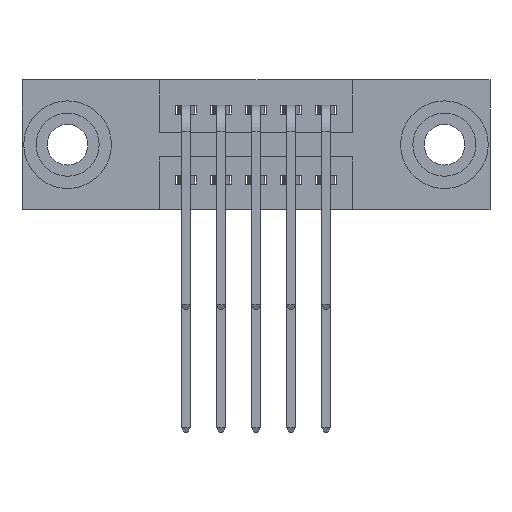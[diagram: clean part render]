
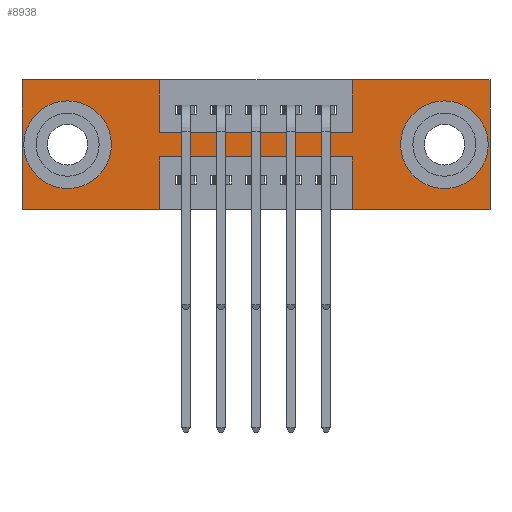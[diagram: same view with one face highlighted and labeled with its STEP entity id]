
A CAD part, front view. The second image highlights one B-rep face of the part: STEP entity #8938.
In plain terms, the highlighted planar face has unit normal (0, -1, 0).
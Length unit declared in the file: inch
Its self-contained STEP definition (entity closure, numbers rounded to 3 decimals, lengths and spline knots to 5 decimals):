
#132 = VECTOR ( 'NONE', #8937, 39.37008 ) ;
#180 = CARTESIAN_POINT ( 'NONE',  ( 0.13, 0., -0.107 ) ) ;
#190 = VERTEX_POINT ( 'NONE', #2204 ) ;
#202 = ORIENTED_EDGE ( 'NONE', *, *, #2390, .F. ) ;
#289 = LINE ( 'NONE', #6771, #3451 ) ;
#338 = CARTESIAN_POINT ( 'NONE',  ( 1.205, 0., -0.263 ) ) ;
#362 = VECTOR ( 'NONE', #2451, 39.37008 ) ;
#378 = EDGE_LOOP ( 'NONE', ( #10536, #8988 ) ) ;
#454 = CARTESIAN_POINT ( 'NONE',  ( 0.3925, 0., 0. ) ) ;
#638 = EDGE_CURVE ( 'NONE', #7686, #3815, #10066, .T. ) ;
#700 = LINE ( 'NONE', #9389, #9630 ) ;
#830 = CARTESIAN_POINT ( 'NONE',  ( 1.205, 0., -0.185 ) ) ;
#831 = LINE ( 'NONE', #9449, #10295 ) ;
#842 = EDGE_CURVE ( 'NONE', #7530, #3438, #9108, .T. ) ;
#853 = DIRECTION ( 'NONE',  ( -1., 0., 0. ) ) ;
#1065 = LINE ( 'NONE', #1571, #362 ) ;
#1109 = VERTEX_POINT ( 'NONE', #6565 ) ;
#1244 = VECTOR ( 'NONE', #3058, 39.37008 ) ;
#1246 = ORIENTED_EDGE ( 'NONE', *, *, #2250, .T. ) ;
#1366 = DIRECTION ( 'NONE',  ( 0., 1., 0. ) ) ;
#1538 = EDGE_CURVE ( 'NONE', #1109, #5867, #289, .T. ) ;
#1571 = CARTESIAN_POINT ( 'NONE',  ( 0., 0., 0. ) ) ;
#1738 = CARTESIAN_POINT ( 'NONE',  ( 0., 0., 0. ) ) ;
#1901 = EDGE_CURVE ( 'NONE', #7118, #190, #700, .T. ) ;
#1912 = CARTESIAN_POINT ( 'NONE',  ( 0.3925, 0., 0. ) ) ;
#2017 = AXIS2_PLACEMENT_3D ( 'NONE', #9764, #1366, #9196 ) ;
#2029 = CIRCLE ( 'NONE', #9321, 0.078 ) ;
#2113 = CARTESIAN_POINT ( 'NONE',  ( 0.3925, 0., -0.15 ) ) ;
#2202 = EDGE_CURVE ( 'NONE', #190, #5864, #2765, .T. ) ;
#2204 = CARTESIAN_POINT ( 'NONE',  ( 0.9425, 0., -0.37 ) ) ;
#2250 = EDGE_CURVE ( 'NONE', #8171, #9735, #3014, .T. ) ;
#2390 = EDGE_CURVE ( 'NONE', #4055, #7118, #831, .T. ) ;
#2399 = CARTESIAN_POINT ( 'NONE',  ( 0., 0., 0. ) ) ;
#2451 = DIRECTION ( 'NONE',  ( 1., 0., 0. ) ) ;
#2468 = DIRECTION ( 'NONE',  ( 0., 1., 0. ) ) ;
#2560 = FACE_OUTER_BOUND ( 'NONE', #3267, .T. ) ;
#2689 = VECTOR ( 'NONE', #5883, 39.37008 ) ;
#2765 = LINE ( 'NONE', #6328, #132 ) ;
#2874 = CARTESIAN_POINT ( 'NONE',  ( 0.3925, 0., -0.22 ) ) ;
#2914 = CARTESIAN_POINT ( 'NONE',  ( 0.3925, 0., -0.15 ) ) ;
#3014 = CIRCLE ( 'NONE', #3895, 0.078 ) ;
#3042 = CARTESIAN_POINT ( 'NONE',  ( 0., 0., -0.37 ) ) ;
#3047 = ORIENTED_EDGE ( 'NONE', *, *, #638, .F. ) ;
#3054 = CARTESIAN_POINT ( 'NONE',  ( 0.3925, 0., -0.22 ) ) ;
#3058 = DIRECTION ( 'NONE',  ( 1., 0., 0. ) ) ;
#3183 = VERTEX_POINT ( 'NONE', #2914 ) ;
#3197 = DIRECTION ( 'NONE',  ( -1., 0., 0. ) ) ;
#3214 = EDGE_CURVE ( 'NONE', #5265, #10917, #5685, .T. ) ;
#3267 = EDGE_LOOP ( 'NONE', ( #3047, #7719, #7498, #3424, #202, #5634, #7673, #6464, #8298, #10031, #10644, #8394 ) ) ;
#3424 = ORIENTED_EDGE ( 'NONE', *, *, #1901, .F. ) ;
#3438 = VERTEX_POINT ( 'NONE', #338 ) ;
#3451 = VECTOR ( 'NONE', #5842, 39.37008 ) ;
#3535 = EDGE_CURVE ( 'NONE', #3807, #3183, #10944, .T. ) ;
#3540 = VECTOR ( 'NONE', #8342, 39.37008 ) ;
#3636 = CARTESIAN_POINT ( 'NONE',  ( 0.13, 0., -0.185 ) ) ;
#3680 = ORIENTED_EDGE ( 'NONE', *, *, #3994, .T. ) ;
#3701 = EDGE_CURVE ( 'NONE', #5867, #4055, #1065, .T. ) ;
#3708 = DIRECTION ( 'NONE',  ( 0., 1., 0. ) ) ;
#3807 = VERTEX_POINT ( 'NONE', #1912 ) ;
#3815 = VERTEX_POINT ( 'NONE', #5576 ) ;
#3895 = AXIS2_PLACEMENT_3D ( 'NONE', #7612, #2468, #5875 ) ;
#3994 = EDGE_CURVE ( 'NONE', #9735, #8171, #2029, .T. ) ;
#4020 = CARTESIAN_POINT ( 'NONE',  ( 0.3925, 0., -0.37 ) ) ;
#4055 = VERTEX_POINT ( 'NONE', #9660 ) ;
#4200 = DIRECTION ( 'NONE',  ( 0., 1., 0. ) ) ;
#4464 = LINE ( 'NONE', #6498, #10279 ) ;
#4509 = AXIS2_PLACEMENT_3D ( 'NONE', #3042, #4632, #10741 ) ;
#4632 = DIRECTION ( 'NONE',  ( 0., -1., 0. ) ) ;
#5265 = VERTEX_POINT ( 'NONE', #6863 ) ;
#5469 = VECTOR ( 'NONE', #5832, 39.37008 ) ;
#5576 = CARTESIAN_POINT ( 'NONE',  ( 0.3925, 0., -0.37 ) ) ;
#5630 = EDGE_CURVE ( 'NONE', #3183, #1109, #10305, .T. ) ;
#5634 = ORIENTED_EDGE ( 'NONE', *, *, #3701, .F. ) ;
#5685 = LINE ( 'NONE', #10138, #10539 ) ;
#5832 = DIRECTION ( 'NONE',  ( 0., 0., -1. ) ) ;
#5842 = DIRECTION ( 'NONE',  ( 0., 0., 1. ) ) ;
#5864 = VERTEX_POINT ( 'NONE', #7512 ) ;
#5867 = VERTEX_POINT ( 'NONE', #6929 ) ;
#5875 = DIRECTION ( 'NONE',  ( 0., 0., 1. ) ) ;
#5876 = DIRECTION ( 'NONE',  ( 0., 0., -1. ) ) ;
#5883 = DIRECTION ( 'NONE',  ( 1., 0., 0. ) ) ;
#6102 = EDGE_CURVE ( 'NONE', #3438, #7530, #10172, .T. ) ;
#6198 = DIRECTION ( 'NONE',  ( 0., 0., 1. ) ) ;
#6328 = CARTESIAN_POINT ( 'NONE',  ( 0.9425, 0., -0.37 ) ) ;
#6416 = AXIS2_PLACEMENT_3D ( 'NONE', #830, #4200, #5876 ) ;
#6464 = ORIENTED_EDGE ( 'NONE', *, *, #5630, .F. ) ;
#6498 = CARTESIAN_POINT ( 'NONE',  ( 0., 0., -0.37 ) ) ;
#6565 = CARTESIAN_POINT ( 'NONE',  ( 0.9425, 0., -0.15 ) ) ;
#6771 = CARTESIAN_POINT ( 'NONE',  ( 0.9425, 0., 0. ) ) ;
#6863 = CARTESIAN_POINT ( 'NONE',  ( 0., 0., -0.37 ) ) ;
#6929 = CARTESIAN_POINT ( 'NONE',  ( 0.9425, 0., 0. ) ) ;
#7099 = CARTESIAN_POINT ( 'NONE',  ( 1.205, 0., -0.107 ) ) ;
#7118 = VERTEX_POINT ( 'NONE', #7884 ) ;
#7195 = PLANE ( 'NONE',  #4509 ) ;
#7261 = FACE_BOUND ( 'NONE', #10288, .T. ) ;
#7498 = ORIENTED_EDGE ( 'NONE', *, *, #2202, .F. ) ;
#7512 = CARTESIAN_POINT ( 'NONE',  ( 0.9425, 0., -0.22 ) ) ;
#7530 = VERTEX_POINT ( 'NONE', #7099 ) ;
#7612 = CARTESIAN_POINT ( 'NONE',  ( 0.13, 0., -0.185 ) ) ;
#7673 = ORIENTED_EDGE ( 'NONE', *, *, #1538, .F. ) ;
#7686 = VERTEX_POINT ( 'NONE', #2874 ) ;
#7719 = ORIENTED_EDGE ( 'NONE', *, *, #8455, .F. ) ;
#7773 = LINE ( 'NONE', #2399, #2689 ) ;
#7802 = EDGE_CURVE ( 'NONE', #3815, #5265, #4464, .T. ) ;
#7884 = CARTESIAN_POINT ( 'NONE',  ( 1.335, 0., -0.37 ) ) ;
#7948 = LINE ( 'NONE', #3054, #9182 ) ;
#8171 = VERTEX_POINT ( 'NONE', #180 ) ;
#8298 = ORIENTED_EDGE ( 'NONE', *, *, #3535, .F. ) ;
#8342 = DIRECTION ( 'NONE',  ( 0., 0., -1. ) ) ;
#8394 = ORIENTED_EDGE ( 'NONE', *, *, #7802, .F. ) ;
#8455 = EDGE_CURVE ( 'NONE', #5864, #7686, #7948, .T. ) ;
#8937 = DIRECTION ( 'NONE',  ( 0., 0., 1. ) ) ;
#8938 = ADVANCED_FACE ( 'NONE', ( #9571, #7261, #2560 ), #7195, .T. ) ;
#8988 = ORIENTED_EDGE ( 'NONE', *, *, #6102, .T. ) ;
#9108 = CIRCLE ( 'NONE', #6416, 0.078 ) ;
#9182 = VECTOR ( 'NONE', #10914, 39.37008 ) ;
#9196 = DIRECTION ( 'NONE',  ( 0., 0., -1. ) ) ;
#9321 = AXIS2_PLACEMENT_3D ( 'NONE', #3636, #3708, #6198 ) ;
#9389 = CARTESIAN_POINT ( 'NONE',  ( 0., 0., -0.37 ) ) ;
#9409 = DIRECTION ( 'NONE',  ( 0., 0., -1. ) ) ;
#9449 = CARTESIAN_POINT ( 'NONE',  ( 1.335, 0., 0. ) ) ;
#9571 = FACE_BOUND ( 'NONE', #378, .T. ) ;
#9630 = VECTOR ( 'NONE', #853, 39.37008 ) ;
#9660 = CARTESIAN_POINT ( 'NONE',  ( 1.335, 0., 0. ) ) ;
#9735 = VERTEX_POINT ( 'NONE', #10924 ) ;
#9754 = EDGE_CURVE ( 'NONE', #10917, #3807, #7773, .T. ) ;
#9764 = CARTESIAN_POINT ( 'NONE',  ( 1.205, 0., -0.185 ) ) ;
#10031 = ORIENTED_EDGE ( 'NONE', *, *, #9754, .F. ) ;
#10066 = LINE ( 'NONE', #4020, #5469 ) ;
#10138 = CARTESIAN_POINT ( 'NONE',  ( 0., 0., 0. ) ) ;
#10172 = CIRCLE ( 'NONE', #2017, 0.078 ) ;
#10208 = DIRECTION ( 'NONE',  ( 0., 0., 1. ) ) ;
#10279 = VECTOR ( 'NONE', #3197, 39.37008 ) ;
#10288 = EDGE_LOOP ( 'NONE', ( #1246, #3680 ) ) ;
#10295 = VECTOR ( 'NONE', #9409, 39.37008 ) ;
#10305 = LINE ( 'NONE', #2113, #1244 ) ;
#10536 = ORIENTED_EDGE ( 'NONE', *, *, #842, .T. ) ;
#10539 = VECTOR ( 'NONE', #10208, 39.37008 ) ;
#10644 = ORIENTED_EDGE ( 'NONE', *, *, #3214, .F. ) ;
#10741 = DIRECTION ( 'NONE',  ( 0., 0., -1. ) ) ;
#10914 = DIRECTION ( 'NONE',  ( -1., 0., 0. ) ) ;
#10917 = VERTEX_POINT ( 'NONE', #1738 ) ;
#10924 = CARTESIAN_POINT ( 'NONE',  ( 0.13, 0., -0.263 ) ) ;
#10944 = LINE ( 'NONE', #454, #3540 ) ;
